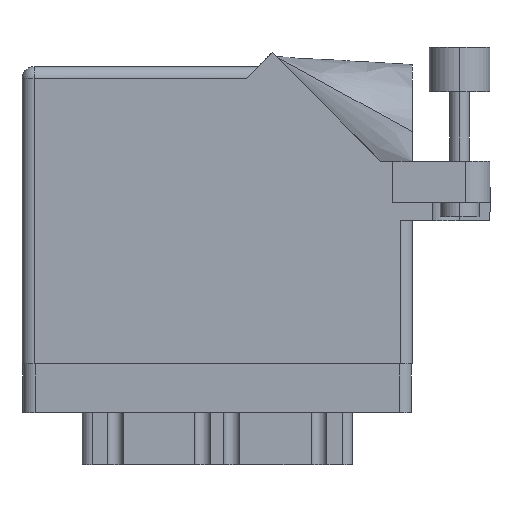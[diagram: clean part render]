
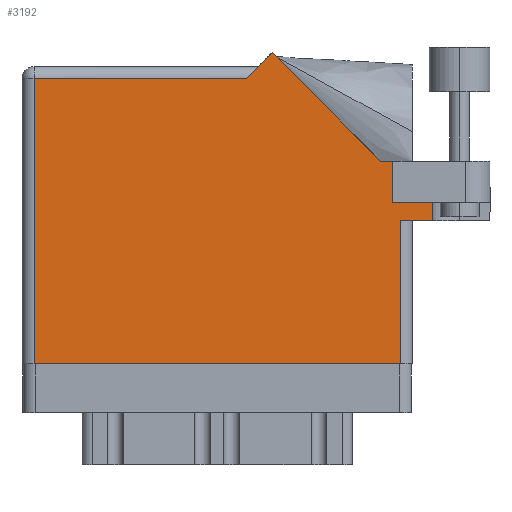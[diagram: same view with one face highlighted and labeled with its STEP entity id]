
A CAD part, front view. The second image highlights one B-rep face of the part: STEP entity #3192.
In plain terms, the highlighted face is planar.
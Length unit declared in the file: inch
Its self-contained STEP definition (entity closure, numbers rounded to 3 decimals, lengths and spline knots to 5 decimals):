
#958 = EDGE_CURVE ( 'NONE', #8630, #4301, #10364, .T. ) ;
#970 = DIRECTION ( 'NONE',  ( 1., 0., 0. ) ) ;
#1265 = CARTESIAN_POINT ( 'NONE',  ( 1.948, 0., 0. ) ) ;
#2920 = CARTESIAN_POINT ( 'NONE',  ( 1.91, 0.831, 0. ) ) ;
#3192 = ADVANCED_FACE ( 'NONE', ( #20093 ), #17406, .F. ) ;
#3293 = ORIENTED_EDGE ( 'NONE', *, *, #17532, .T. ) ;
#3332 = CARTESIAN_POINT ( 'NONE',  ( 2.41, 1.044, 0. ) ) ;
#3658 = LINE ( 'NONE', #28274, #27315 ) ;
#4001 = EDGE_LOOP ( 'NONE', ( #16488, #19490, #32883, #14135, #30009, #19635, #31443, #18950, #3293, #12535, #22248 ) ) ;
#4287 = VECTOR ( 'NONE', #32115, 39.37008 ) ;
#4301 = VERTEX_POINT ( 'NONE', #25968 ) ;
#5439 = VERTEX_POINT ( 'NONE', #5999 ) ;
#5951 = VERTEX_POINT ( 'NONE', #16317 ) ;
#5999 = CARTESIAN_POINT ( 'NONE',  ( 1.91, 1.044, 0. ) ) ;
#6896 = VECTOR ( 'NONE', #30635, 39.37008 ) ;
#7045 = VECTOR ( 'NONE', #29750, 39.37008 ) ;
#7654 = DIRECTION ( 'NONE',  ( -0.707, -0.707, 0. ) ) ;
#7984 = CARTESIAN_POINT ( 'NONE',  ( 1.948, 0.737, 0. ) ) ;
#8630 = VERTEX_POINT ( 'NONE', #26789 ) ;
#8890 = DIRECTION ( 'NONE',  ( 0., -1., 0. ) ) ;
#9236 = VERTEX_POINT ( 'NONE', #19917 ) ;
#9409 = LINE ( 'NONE', #28146, #6896 ) ;
#9915 = CARTESIAN_POINT ( 'NONE',  ( 1.28771, 1.60071, 0. ) ) ;
#10197 = LINE ( 'NONE', #18586, #27784 ) ;
#10260 = EDGE_CURVE ( 'NONE', #9236, #22911, #31560, .T. ) ;
#10364 = LINE ( 'NONE', #21249, #4287 ) ;
#10505 = DIRECTION ( 'NONE',  ( 1., 0., 0. ) ) ;
#10580 = EDGE_CURVE ( 'NONE', #4301, #5951, #25666, .T. ) ;
#12535 = ORIENTED_EDGE ( 'NONE', *, *, #958, .T. ) ;
#12699 = EDGE_CURVE ( 'NONE', #5951, #16621, #9409, .T. ) ;
#13916 = CARTESIAN_POINT ( 'NONE',  ( 1.91, 0.831, 0. ) ) ;
#14016 = LINE ( 'NONE', #3332, #30203 ) ;
#14135 = ORIENTED_EDGE ( 'NONE', *, *, #24584, .F. ) ;
#14355 = EDGE_CURVE ( 'NONE', #31780, #26621, #3658, .T. ) ;
#16317 = CARTESIAN_POINT ( 'NONE',  ( 0.062, 0., 0. ) ) ;
#16488 = ORIENTED_EDGE ( 'NONE', *, *, #12699, .T. ) ;
#16621 = VERTEX_POINT ( 'NONE', #1265 ) ;
#16834 = VECTOR ( 'NONE', #10505, 39.37008 ) ;
#17184 = CARTESIAN_POINT ( 'NONE',  ( 1.91, 0.831, 0. ) ) ;
#17406 = PLANE ( 'NONE',  #26715 ) ;
#17532 = EDGE_CURVE ( 'NONE', #26621, #8630, #23908, .T. ) ;
#18586 = CARTESIAN_POINT ( 'NONE',  ( 2.1115, 1.16177, 0. ) ) ;
#18880 = LINE ( 'NONE', #7984, #7045 ) ;
#18950 = ORIENTED_EDGE ( 'NONE', *, *, #14355, .T. ) ;
#19098 = EDGE_CURVE ( 'NONE', #20957, #5439, #33395, .T. ) ;
#19490 = ORIENTED_EDGE ( 'NONE', *, *, #21117, .T. ) ;
#19635 = ORIENTED_EDGE ( 'NONE', *, *, #19098, .T. ) ;
#19917 = CARTESIAN_POINT ( 'NONE',  ( 1.948, 0.737, 0. ) ) ;
#20093 = FACE_OUTER_BOUND ( 'NONE', #4001, .T. ) ;
#20717 = CARTESIAN_POINT ( 'NONE',  ( 2.1115, 0.831, 0. ) ) ;
#20957 = VERTEX_POINT ( 'NONE', #13916 ) ;
#21051 = CARTESIAN_POINT ( 'NONE',  ( 1.217, 1.53, 0. ) ) ;
#21117 = EDGE_CURVE ( 'NONE', #16621, #9236, #18880, .T. ) ;
#21249 = CARTESIAN_POINT ( 'NONE',  ( 0., 1.468, 0. ) ) ;
#22248 = ORIENTED_EDGE ( 'NONE', *, *, #10580, .T. ) ;
#22835 = VECTOR ( 'NONE', #970, 39.37008 ) ;
#22911 = VERTEX_POINT ( 'NONE', #29314 ) ;
#23908 = LINE ( 'NONE', #21051, #33639 ) ;
#24556 = DIRECTION ( 'NONE',  ( -1., 0., 0. ) ) ;
#24584 = EDGE_CURVE ( 'NONE', #32392, #22911, #10197, .T. ) ;
#25666 = LINE ( 'NONE', #33159, #32995 ) ;
#25968 = CARTESIAN_POINT ( 'NONE',  ( 0.062, 1.468, 0. ) ) ;
#26621 = VERTEX_POINT ( 'NONE', #9915 ) ;
#26715 = AXIS2_PLACEMENT_3D ( 'NONE', #33811, #32612, #27441 ) ;
#26789 = CARTESIAN_POINT ( 'NONE',  ( 1.155, 1.468, 0. ) ) ;
#27315 = VECTOR ( 'NONE', #27734, 39.37008 ) ;
#27441 = DIRECTION ( 'NONE',  ( -1., 0., 0. ) ) ;
#27734 = DIRECTION ( 'NONE',  ( -0.707, 0.707, 0. ) ) ;
#27784 = VECTOR ( 'NONE', #34290, 39.37008 ) ;
#28042 = EDGE_CURVE ( 'NONE', #5439, #31780, #14016, .T. ) ;
#28146 = CARTESIAN_POINT ( 'NONE',  ( 0., 0., 0. ) ) ;
#28274 = CARTESIAN_POINT ( 'NONE',  ( 1.84442, 1.044, 0. ) ) ;
#28567 = EDGE_CURVE ( 'NONE', #20957, #32392, #30556, .T. ) ;
#28861 = CARTESIAN_POINT ( 'NONE',  ( 1.84442, 1.044, 0. ) ) ;
#29314 = CARTESIAN_POINT ( 'NONE',  ( 2.1115, 0.737, 0. ) ) ;
#29750 = DIRECTION ( 'NONE',  ( 0., 1., 0. ) ) ;
#30009 = ORIENTED_EDGE ( 'NONE', *, *, #28567, .F. ) ;
#30203 = VECTOR ( 'NONE', #24556, 39.37008 ) ;
#30556 = LINE ( 'NONE', #17184, #22835 ) ;
#30635 = DIRECTION ( 'NONE',  ( 1., 0., 0. ) ) ;
#31443 = ORIENTED_EDGE ( 'NONE', *, *, #28042, .T. ) ;
#31560 = LINE ( 'NONE', #32086, #16834 ) ;
#31780 = VERTEX_POINT ( 'NONE', #28861 ) ;
#32086 = CARTESIAN_POINT ( 'NONE',  ( 2.01, 0.737, 0. ) ) ;
#32115 = DIRECTION ( 'NONE',  ( -1., 0., 0. ) ) ;
#32392 = VERTEX_POINT ( 'NONE', #20717 ) ;
#32612 = DIRECTION ( 'NONE',  ( 0., 0., -1. ) ) ;
#32883 = ORIENTED_EDGE ( 'NONE', *, *, #10260, .T. ) ;
#32995 = VECTOR ( 'NONE', #8890, 39.37008 ) ;
#33036 = DIRECTION ( 'NONE',  ( 0., 1., 0. ) ) ;
#33159 = CARTESIAN_POINT ( 'NONE',  ( 0.062, 0., 0. ) ) ;
#33395 = LINE ( 'NONE', #2920, #33713 ) ;
#33639 = VECTOR ( 'NONE', #7654, 39.37008 ) ;
#33713 = VECTOR ( 'NONE', #33036, 39.37008 ) ;
#33811 = CARTESIAN_POINT ( 'NONE',  ( 0., 1.53, 0. ) ) ;
#34290 = DIRECTION ( 'NONE',  ( 0., -1., 0. ) ) ;
